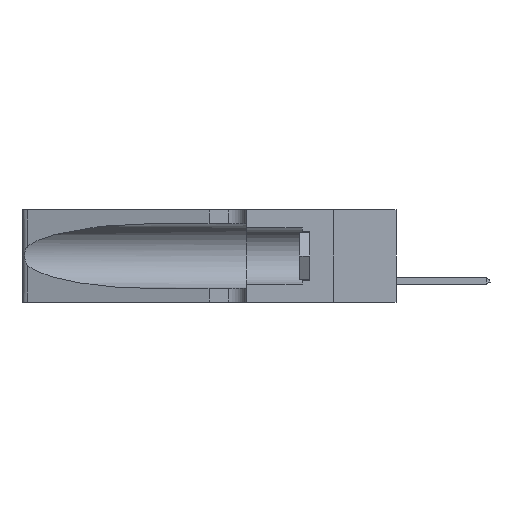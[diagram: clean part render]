
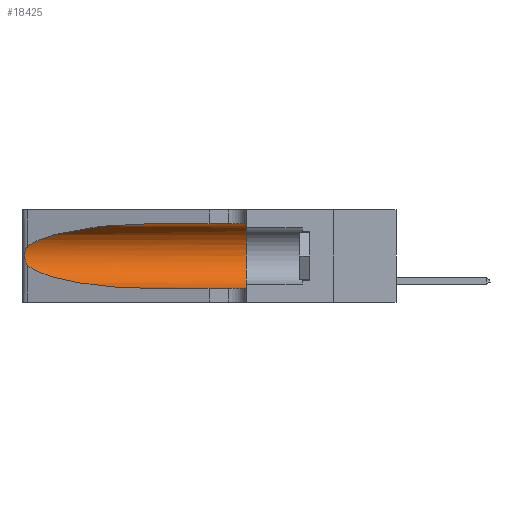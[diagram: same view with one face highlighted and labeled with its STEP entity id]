
A CAD part, left-side view. The second image highlights one B-rep face of the part: STEP entity #18425.
In plain terms, the highlighted cylindrical face has radius 3.308 mm (diameter 6.617 mm), a partial arc.
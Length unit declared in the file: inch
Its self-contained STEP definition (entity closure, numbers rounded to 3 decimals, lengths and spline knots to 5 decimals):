
#851 = CARTESIAN_POINT ( 'NONE',  ( 0.25639, 1.23186, 0.15144 ) ) ;
#1159 = CARTESIAN_POINT ( 'NONE',  ( 0.26075, 1.23896, 0.19203 ) ) ;
#1815 = VERTEX_POINT ( 'NONE', #21885 ) ;
#2473 = EDGE_CURVE ( 'NONE', #24369, #29398, #30728, .T. ) ;
#3342 =( BOUNDED_CURVE ( )  B_SPLINE_CURVE ( 3, ( #8173, #10404, #25043, #7954 ),
 .UNSPECIFIED., .F., .F. ) 
 B_SPLINE_CURVE_WITH_KNOTS ( ( 4, 4 ),
 ( 3.44316, 4.71239 ),
 .UNSPECIFIED. ) 
 CURVE ( )  GEOMETRIC_REPRESENTATION_ITEM ( )  RATIONAL_B_SPLINE_CURVE ( ( 1., 0.87, 0.87, 1. ) ) 
 REPRESENTATION_ITEM ( '' )  );
#3920 = EDGE_LOOP ( 'NONE', ( #10993, #7263, #18198, #13480, #26883, #16608 ) ) ;
#5169 = CARTESIAN_POINT ( 'NONE',  ( 0.1305, 0.35, 0.185 ) ) ;
#5248 = EDGE_CURVE ( 'NONE', #1815, #24369, #27734, .T. ) ;
#5836 = CARTESIAN_POINT ( 'NONE',  ( 0.25789, 1.23486, 0.15765 ) ) ;
#5954 = CARTESIAN_POINT ( 'NONE',  ( 0.25854, 1.2359, 0.20912 ) ) ;
#7228 = CARTESIAN_POINT ( 'NONE',  ( 0.18966, 0.96281, 0.31525 ) ) ;
#7263 = ORIENTED_EDGE ( 'NONE', *, *, #20174, .T. ) ;
#7954 = CARTESIAN_POINT ( 'NONE',  ( 0.1305, 0.72297, 0.05475 ) ) ;
#8098 = CARTESIAN_POINT ( 'NONE',  ( 0.1305, 1.61858, 0.31525 ) ) ;
#8173 = CARTESIAN_POINT ( 'NONE',  ( 0.25487, 1.22718, 0.14631 ) ) ;
#8286 = CARTESIAN_POINT ( 'NONE',  ( 0.25787, 1.23484, 0.2124 ) ) ;
#8327 = DIRECTION ( 'NONE',  ( 0., 0., 1. ) ) ;
#8481 = VECTOR ( 'NONE', #29720, 39.37008 ) ;
#8511 = CARTESIAN_POINT ( 'NONE',  ( 0.25639, 1.23184, 0.21858 ) ) ;
#8950 = LINE ( 'NONE', #14072, #27432 ) ;
#9028 = VERTEX_POINT ( 'NONE', #21811 ) ;
#9300 = AXIS2_PLACEMENT_3D ( 'NONE', #30152, #25411, #27632 ) ;
#10404 = CARTESIAN_POINT ( 'NONE',  ( 0.2373, 1.15595, 0.08982 ) ) ;
#10622 = CARTESIAN_POINT ( 'NONE',  ( 0.25487, 1.22718, 0.14631 ) ) ;
#10993 = ORIENTED_EDGE ( 'NONE', *, *, #11694, .T. ) ;
#11694 = EDGE_CURVE ( 'NONE', #1815, #9028, #23117, .T. ) ;
#13480 = ORIENTED_EDGE ( 'NONE', *, *, #31043, .T. ) ;
#14072 = CARTESIAN_POINT ( 'NONE',  ( 0.1305, 1.61858, 0.05475 ) ) ;
#14103 = CARTESIAN_POINT ( 'NONE',  ( 0.1305, 0.35, 0.05475 ) ) ;
#16608 = ORIENTED_EDGE ( 'NONE', *, *, #5248, .F. ) ;
#17757 = CARTESIAN_POINT ( 'NONE',  ( 0.1305, 0.72297, 0.05475 ) ) ;
#17859 = VERTEX_POINT ( 'NONE', #21956 ) ;
#17871 = CARTESIAN_POINT ( 'NONE',  ( 0.25555, 1.22993, 0.14849 ) ) ;
#18198 = ORIENTED_EDGE ( 'NONE', *, *, #28333, .T. ) ;
#18425 = ADVANCED_FACE ( 'NONE', ( #26131 ), #28004, .F. ) ;
#20174 = EDGE_CURVE ( 'NONE', #9028, #17859, #25026, .T. ) ;
#21811 = CARTESIAN_POINT ( 'NONE',  ( 0.25487, 1.22718, 0.22369 ) ) ;
#21885 = CARTESIAN_POINT ( 'NONE',  ( 0.1305, 0.72297, 0.31525 ) ) ;
#21948 = VERTEX_POINT ( 'NONE', #17757 ) ;
#21956 = CARTESIAN_POINT ( 'NONE',  ( 0.25487, 1.22718, 0.14631 ) ) ;
#22887 = CARTESIAN_POINT ( 'NONE',  ( 0.25487, 1.22718, 0.22369 ) ) ;
#22963 = CARTESIAN_POINT ( 'NONE',  ( 0.25555, 1.22994, 0.2215 ) ) ;
#23117 =( BOUNDED_CURVE ( )  B_SPLINE_CURVE ( 3, ( #23882, #7228, #27639, #22887 ),
 .UNSPECIFIED., .F., .F. ) 
 B_SPLINE_CURVE_WITH_KNOTS ( ( 4, 4 ),
 ( 1.5708, 2.84003 ),
 .UNSPECIFIED. ) 
 CURVE ( )  GEOMETRIC_REPRESENTATION_ITEM ( )  RATIONAL_B_SPLINE_CURVE ( ( 1., 0.87, 0.87, 1. ) ) 
 REPRESENTATION_ITEM ( '' )  );
#23882 = CARTESIAN_POINT ( 'NONE',  ( 0.1305, 0.72297, 0.31525 ) ) ;
#24369 = VERTEX_POINT ( 'NONE', #29427 ) ;
#24953 = CARTESIAN_POINT ( 'NONE',  ( 0.25856, 1.23593, 0.16098 ) ) ;
#25026 = B_SPLINE_CURVE_WITH_KNOTS ( 'NONE', 3,
 ( #29886, #22963, #8511, #8286, #5954, #27602, #1159, #25173, #30127, #24953, #5836, #851, #17871, #10622 ),
 .UNSPECIFIED., .F., .F.,
 ( 4, 2, 2, 2, 2, 2, 4 ),
 ( 0., 0.00027, 0.00053, 0.00107, 0.0016, 0.00187, 0.00214 ),
 .UNSPECIFIED. ) ;
#25043 = CARTESIAN_POINT ( 'NONE',  ( 0.18966, 0.96281, 0.05475 ) ) ;
#25173 = CARTESIAN_POINT ( 'NONE',  ( 0.26075, 1.23896, 0.178 ) ) ;
#25411 = DIRECTION ( 'NONE',  ( 0., -1., 0. ) ) ;
#26131 = FACE_OUTER_BOUND ( 'NONE', #3920, .T. ) ;
#26883 = ORIENTED_EDGE ( 'NONE', *, *, #2473, .F. ) ;
#27432 = VECTOR ( 'NONE', #28680, 39.37008 ) ;
#27602 = CARTESIAN_POINT ( 'NONE',  ( 0.26018, 1.23835, 0.19895 ) ) ;
#27632 = DIRECTION ( 'NONE',  ( 0., 0., -1. ) ) ;
#27639 = CARTESIAN_POINT ( 'NONE',  ( 0.2373, 1.15595, 0.28018 ) ) ;
#27734 = LINE ( 'NONE', #8098, #8481 ) ;
#28004 = CYLINDRICAL_SURFACE ( 'NONE', #9300, 0.13025 ) ;
#28333 = EDGE_CURVE ( 'NONE', #17859, #21948, #3342, .T. ) ;
#28680 = DIRECTION ( 'NONE',  ( 0., -1., 0. ) ) ;
#29317 = DIRECTION ( 'NONE',  ( 0., 1., 0. ) ) ;
#29398 = VERTEX_POINT ( 'NONE', #14103 ) ;
#29427 = CARTESIAN_POINT ( 'NONE',  ( 0.1305, 0.35, 0.31525 ) ) ;
#29720 = DIRECTION ( 'NONE',  ( 0., -1., 0. ) ) ;
#29886 = CARTESIAN_POINT ( 'NONE',  ( 0.25487, 1.22718, 0.22369 ) ) ;
#30127 = CARTESIAN_POINT ( 'NONE',  ( 0.26017, 1.23833, 0.17102 ) ) ;
#30152 = CARTESIAN_POINT ( 'NONE',  ( 0.1305, 1.61858, 0.185 ) ) ;
#30722 = AXIS2_PLACEMENT_3D ( 'NONE', #5169, #29317, #8327 ) ;
#30728 = CIRCLE ( 'NONE', #30722, 0.13025 ) ;
#31043 = EDGE_CURVE ( 'NONE', #21948, #29398, #8950, .T. ) ;
